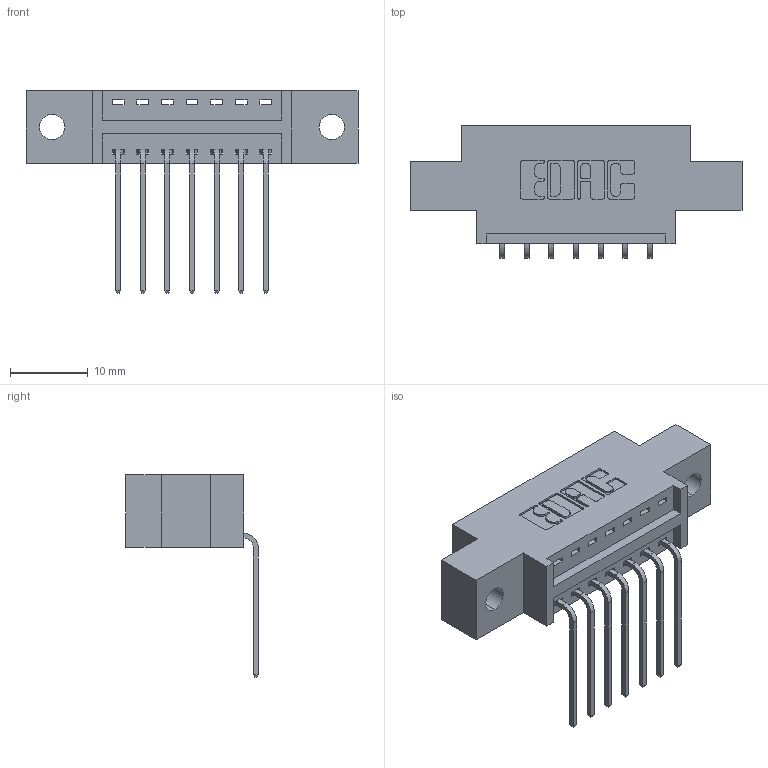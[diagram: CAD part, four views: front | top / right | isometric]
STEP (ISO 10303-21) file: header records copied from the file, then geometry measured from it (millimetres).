
FILE_DESCRIPTION (( 'STEP AP203' ), '1' );
FILE_NAME ('346-007-559-602.STEP', '2018-08-17T04:17:57', ( '' ), ( '' ), 'SwSTEP 2.0', 'SolidWorks 2016', '' );
FILE_SCHEMA (( 'CONFIG_CONTROL_DESIGN' ));
Length unit declared in the file: inch
Products named in the file (3): 346 Part_0.170 Offset - 0.128 Dia; 345-292-001_558 559 Tail - 1; 346-007-559-602
Assembly tree (8 placements, depth 2):
  346-007-559-602
    346 Part_0.170 Offset - 0.128 Dia
    345-292-001_558 559 Tail - 1  x7
Bounding box: 42.8 x 17.08 x 26.16 mm (x, y, z)
Volume: 3687.7 mm3; surface area: 4259.7 mm2
Topology: 8 solids, 8 shells, 546 faces, 1615 edges, 1066 vertices
Faces by surface type: plane 374, cylinder 172
Entity records: 9275 total; most frequent: CARTESIAN_POINT 1609, ORIENTED_EDGE 1550, DIRECTION 1461, EDGE_CURVE 775, VECTOR 615, LINE 615, VERTEX_POINT 514, AXIS2_PLACEMENT_3D 423
